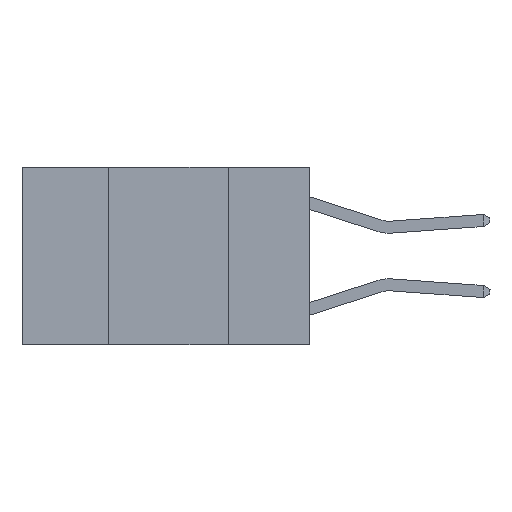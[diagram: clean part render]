
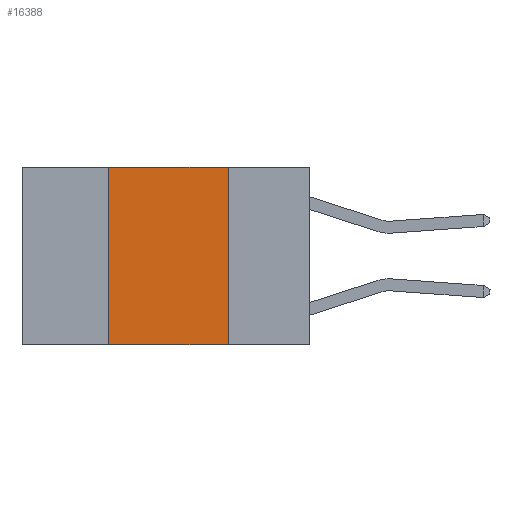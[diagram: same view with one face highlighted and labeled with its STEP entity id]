
A CAD part, left-side view. The second image highlights one B-rep face of the part: STEP entity #16388.
In plain terms, the highlighted planar face has unit normal (-1, 0, 0).
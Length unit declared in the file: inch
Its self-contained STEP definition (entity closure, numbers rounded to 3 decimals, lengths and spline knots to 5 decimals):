
#1228 = VERTEX_POINT ( 'NONE', #6765 ) ;
#2128 = LINE ( 'NONE', #2742, #18321 ) ;
#2742 = CARTESIAN_POINT ( 'NONE',  ( 0., 0.17, 0. ) ) ;
#4324 = CARTESIAN_POINT ( 'NONE',  ( 0., 0.6, 0. ) ) ;
#4350 = AXIS2_PLACEMENT_3D ( 'NONE', #7777, #18720, #9338 ) ;
#4383 = VECTOR ( 'NONE', #15316, 39.37008 ) ;
#4429 = CARTESIAN_POINT ( 'NONE',  ( 0., 0.42, 0. ) ) ;
#4703 = EDGE_LOOP ( 'NONE', ( #19318, #12937, #13341, #8725 ) ) ;
#5258 = EDGE_CURVE ( 'NONE', #14055, #18055, #9661, .T. ) ;
#5989 = DIRECTION ( 'NONE',  ( 0., -1., 0. ) ) ;
#6096 = CARTESIAN_POINT ( 'NONE',  ( 0., 0.17, -0.37 ) ) ;
#6313 = EDGE_CURVE ( 'NONE', #14055, #7906, #8877, .T. ) ;
#6765 = CARTESIAN_POINT ( 'NONE',  ( 0., 0.17, 0. ) ) ;
#6821 = FACE_OUTER_BOUND ( 'NONE', #4703, .T. ) ;
#7777 = CARTESIAN_POINT ( 'NONE',  ( 0., 0.6, 0. ) ) ;
#7906 = VERTEX_POINT ( 'NONE', #4429 ) ;
#8670 = CARTESIAN_POINT ( 'NONE',  ( 0., 0.42, -0.37 ) ) ;
#8705 = CARTESIAN_POINT ( 'NONE',  ( 0., 0.42, 0. ) ) ;
#8725 = ORIENTED_EDGE ( 'NONE', *, *, #5258, .T. ) ;
#8877 = LINE ( 'NONE', #8705, #16723 ) ;
#9140 = CARTESIAN_POINT ( 'NONE',  ( 0., 0.6, -0.37 ) ) ;
#9338 = DIRECTION ( 'NONE',  ( 0., 0., -1. ) ) ;
#9457 = EDGE_CURVE ( 'NONE', #1228, #18055, #2128, .T. ) ;
#9661 = LINE ( 'NONE', #9140, #13826 ) ;
#10275 = DIRECTION ( 'NONE',  ( 0., 0., 1. ) ) ;
#12405 = PLANE ( 'NONE',  #4350 ) ;
#12937 = ORIENTED_EDGE ( 'NONE', *, *, #13535, .F. ) ;
#13341 = ORIENTED_EDGE ( 'NONE', *, *, #6313, .F. ) ;
#13535 = EDGE_CURVE ( 'NONE', #7906, #1228, #16940, .T. ) ;
#13826 = VECTOR ( 'NONE', #5989, 39.37008 ) ;
#14055 = VERTEX_POINT ( 'NONE', #8670 ) ;
#15316 = DIRECTION ( 'NONE',  ( 0., -1., 0. ) ) ;
#15317 = DIRECTION ( 'NONE',  ( 0., 0., -1. ) ) ;
#16388 = ADVANCED_FACE ( 'NONE', ( #6821 ), #12405, .F. ) ;
#16723 = VECTOR ( 'NONE', #10275, 39.37008 ) ;
#16940 = LINE ( 'NONE', #4324, #4383 ) ;
#18055 = VERTEX_POINT ( 'NONE', #6096 ) ;
#18321 = VECTOR ( 'NONE', #15317, 39.37008 ) ;
#18720 = DIRECTION ( 'NONE',  ( 1., 0., 0. ) ) ;
#19318 = ORIENTED_EDGE ( 'NONE', *, *, #9457, .F. ) ;
